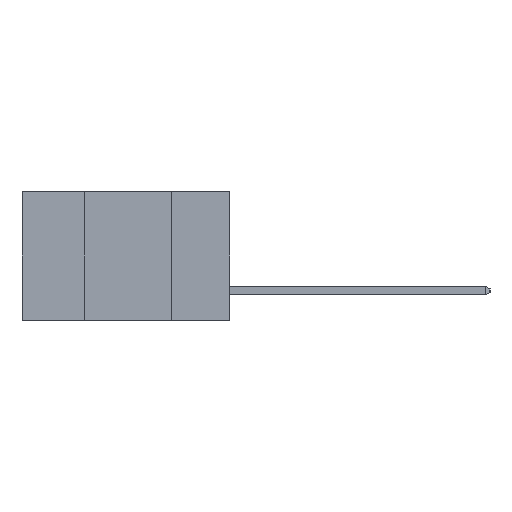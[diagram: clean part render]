
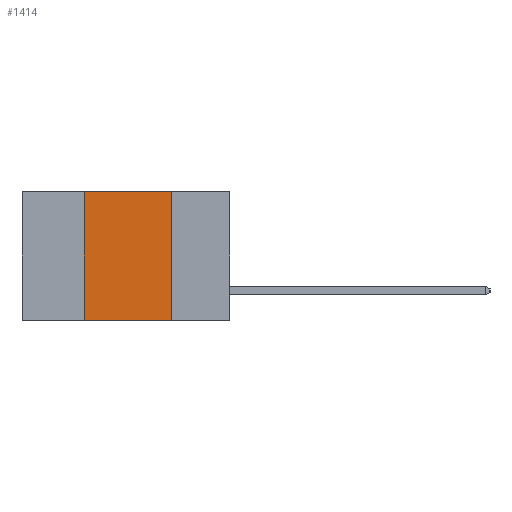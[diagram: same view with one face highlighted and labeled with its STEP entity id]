
A CAD part, left-side view. The second image highlights one B-rep face of the part: STEP entity #1414.
In plain terms, the highlighted planar face has unit normal (-1, 0, 0).
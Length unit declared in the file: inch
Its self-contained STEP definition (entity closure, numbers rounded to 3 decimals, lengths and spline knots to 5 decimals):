
#356 = VERTEX_POINT ( 'NONE', #2378 ) ;
#360 = LINE ( 'NONE', #5472, #3078 ) ;
#580 = CARTESIAN_POINT ( 'NONE',  ( 0., 0.6, -0.37 ) ) ;
#924 = ORIENTED_EDGE ( 'NONE', *, *, #11589, .F. ) ;
#1003 = LINE ( 'NONE', #580, #14886 ) ;
#1103 = EDGE_CURVE ( 'NONE', #14127, #356, #1003, .T. ) ;
#1414 = ADVANCED_FACE ( 'NONE', ( #7106 ), #12974, .F. ) ;
#1497 = VERTEX_POINT ( 'NONE', #14008 ) ;
#1944 = CARTESIAN_POINT ( 'NONE',  ( 0., 0.42, -0.37 ) ) ;
#2049 = DIRECTION ( 'NONE',  ( 0., -1., 0. ) ) ;
#2052 = ORIENTED_EDGE ( 'NONE', *, *, #5310, .F. ) ;
#2167 = DIRECTION ( 'NONE',  ( 0., 0., 1. ) ) ;
#2378 = CARTESIAN_POINT ( 'NONE',  ( 0., 0.17, -0.37 ) ) ;
#2500 = LINE ( 'NONE', #9135, #4672 ) ;
#3078 = VECTOR ( 'NONE', #6718, 39.37008 ) ;
#3567 = DIRECTION ( 'NONE',  ( 1., 0., 0. ) ) ;
#4672 = VECTOR ( 'NONE', #2167, 39.37008 ) ;
#5094 = LINE ( 'NONE', #7903, #5811 ) ;
#5310 = EDGE_CURVE ( 'NONE', #13560, #1497, #5094, .T. ) ;
#5472 = CARTESIAN_POINT ( 'NONE',  ( 0., 0.17, -0.37 ) ) ;
#5811 = VECTOR ( 'NONE', #2049, 39.37008 ) ;
#6043 = CARTESIAN_POINT ( 'NONE',  ( 0., 0.6, 0. ) ) ;
#6050 = EDGE_CURVE ( 'NONE', #1497, #356, #360, .T. ) ;
#6718 = DIRECTION ( 'NONE',  ( 0., 0., -1. ) ) ;
#7106 = FACE_OUTER_BOUND ( 'NONE', #11628, .T. ) ;
#7568 = CARTESIAN_POINT ( 'NONE',  ( 0., 0.42, 0. ) ) ;
#7903 = CARTESIAN_POINT ( 'NONE',  ( 0., 0.6, 0. ) ) ;
#8400 = AXIS2_PLACEMENT_3D ( 'NONE', #6043, #3567, #14143 ) ;
#8575 = DIRECTION ( 'NONE',  ( 0., -1., 0. ) ) ;
#9135 = CARTESIAN_POINT ( 'NONE',  ( 0., 0.42, -0.37 ) ) ;
#9189 = ORIENTED_EDGE ( 'NONE', *, *, #6050, .F. ) ;
#9959 = ORIENTED_EDGE ( 'NONE', *, *, #1103, .T. ) ;
#11589 = EDGE_CURVE ( 'NONE', #14127, #13560, #2500, .T. ) ;
#11628 = EDGE_LOOP ( 'NONE', ( #9189, #2052, #924, #9959 ) ) ;
#12974 = PLANE ( 'NONE',  #8400 ) ;
#13560 = VERTEX_POINT ( 'NONE', #7568 ) ;
#14008 = CARTESIAN_POINT ( 'NONE',  ( 0., 0.17, 0. ) ) ;
#14127 = VERTEX_POINT ( 'NONE', #1944 ) ;
#14143 = DIRECTION ( 'NONE',  ( 0., 0., -1. ) ) ;
#14886 = VECTOR ( 'NONE', #8575, 39.37008 ) ;
